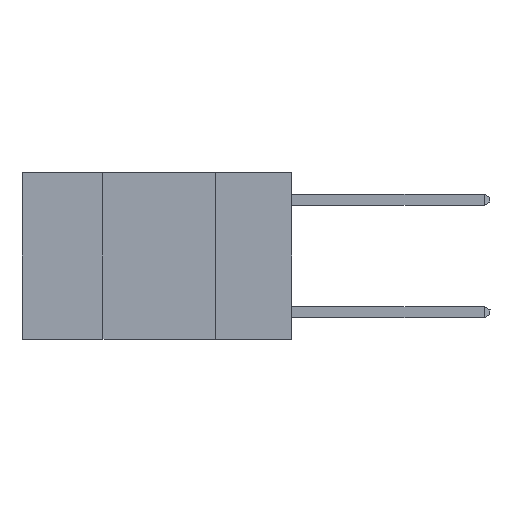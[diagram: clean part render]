
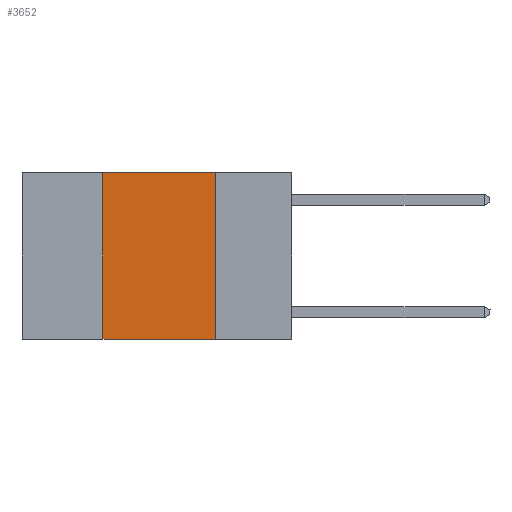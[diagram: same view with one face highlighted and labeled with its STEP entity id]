
A CAD part, left-side view. The second image highlights one B-rep face of the part: STEP entity #3652.
In plain terms, the highlighted planar face has unit normal (-1, 0, 0).
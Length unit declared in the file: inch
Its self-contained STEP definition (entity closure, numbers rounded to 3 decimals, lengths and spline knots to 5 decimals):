
#371 = VERTEX_POINT ( 'NONE', #9210 ) ;
#609 = DIRECTION ( 'NONE',  ( 1., 0., 0. ) ) ;
#883 = LINE ( 'NONE', #12710, #13024 ) ;
#1407 = VERTEX_POINT ( 'NONE', #23394 ) ;
#2068 = AXIS2_PLACEMENT_3D ( 'NONE', #7457, #609, #16423 ) ;
#2686 = FACE_OUTER_BOUND ( 'NONE', #6222, .T. ) ;
#3652 = ADVANCED_FACE ( 'NONE', ( #2686 ), #27259, .F. ) ;
#4434 = EDGE_CURVE ( 'NONE', #371, #13168, #8556, .T. ) ;
#4846 = CARTESIAN_POINT ( 'NONE',  ( 0., 0.42, 0. ) ) ;
#5630 = VECTOR ( 'NONE', #6183, 39.37008 ) ;
#6183 = DIRECTION ( 'NONE',  ( 0., -1., 0. ) ) ;
#6222 = EDGE_LOOP ( 'NONE', ( #28705, #9936, #12581, #12806 ) ) ;
#7085 = DIRECTION ( 'NONE',  ( 0., 0., 1. ) ) ;
#7457 = CARTESIAN_POINT ( 'NONE',  ( 0., 0.6, 0. ) ) ;
#8556 = LINE ( 'NONE', #14165, #25446 ) ;
#9210 = CARTESIAN_POINT ( 'NONE',  ( 0., 0.17, 0. ) ) ;
#9727 = CARTESIAN_POINT ( 'NONE',  ( 0., 0.42, -0.37 ) ) ;
#9936 = ORIENTED_EDGE ( 'NONE', *, *, #11211, .F. ) ;
#10109 = EDGE_CURVE ( 'NONE', #22459, #1407, #18700, .T. ) ;
#11211 = EDGE_CURVE ( 'NONE', #1407, #371, #883, .T. ) ;
#11286 = EDGE_CURVE ( 'NONE', #22459, #13168, #22577, .T. ) ;
#12581 = ORIENTED_EDGE ( 'NONE', *, *, #10109, .F. ) ;
#12710 = CARTESIAN_POINT ( 'NONE',  ( 0., 0.6, 0. ) ) ;
#12806 = ORIENTED_EDGE ( 'NONE', *, *, #11286, .T. ) ;
#13024 = VECTOR ( 'NONE', #19220, 39.37008 ) ;
#13168 = VERTEX_POINT ( 'NONE', #25853 ) ;
#14165 = CARTESIAN_POINT ( 'NONE',  ( 0., 0.17, 0. ) ) ;
#16423 = DIRECTION ( 'NONE',  ( 0., 0., -1. ) ) ;
#18700 = LINE ( 'NONE', #4846, #19394 ) ;
#19220 = DIRECTION ( 'NONE',  ( 0., -1., 0. ) ) ;
#19394 = VECTOR ( 'NONE', #7085, 39.37008 ) ;
#19500 = CARTESIAN_POINT ( 'NONE',  ( 0., 0.6, -0.37 ) ) ;
#22459 = VERTEX_POINT ( 'NONE', #9727 ) ;
#22577 = LINE ( 'NONE', #19500, #5630 ) ;
#23394 = CARTESIAN_POINT ( 'NONE',  ( 0., 0.42, 0. ) ) ;
#25446 = VECTOR ( 'NONE', #27205, 39.37008 ) ;
#25853 = CARTESIAN_POINT ( 'NONE',  ( 0., 0.17, -0.37 ) ) ;
#27205 = DIRECTION ( 'NONE',  ( 0., 0., -1. ) ) ;
#27259 = PLANE ( 'NONE',  #2068 ) ;
#28705 = ORIENTED_EDGE ( 'NONE', *, *, #4434, .F. ) ;
